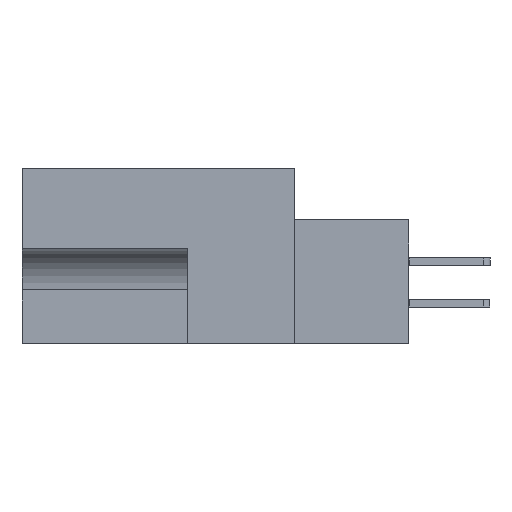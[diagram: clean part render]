
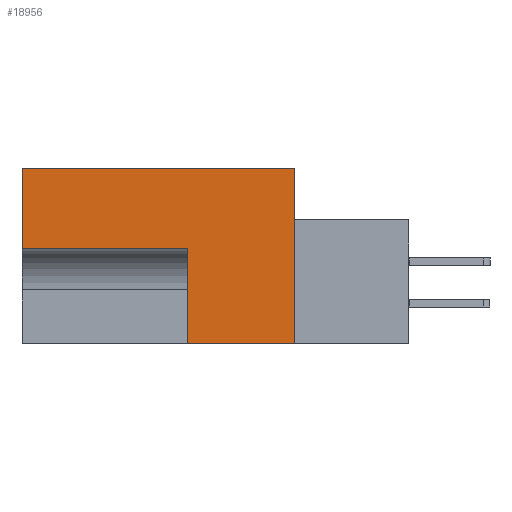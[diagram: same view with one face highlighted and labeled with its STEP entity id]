
A CAD part, left-side view. The second image highlights one B-rep face of the part: STEP entity #18956.
In plain terms, the highlighted planar face has unit normal (-1, 0, 0).
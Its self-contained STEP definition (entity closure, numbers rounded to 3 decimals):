
#2297 = EDGE_CURVE ( 'NONE', #13892, #23138, #31262, .T. ) ;
#3985 = VERTEX_POINT ( 'NONE', #21897 ) ;
#4034 = CARTESIAN_POINT ( 'NONE',  ( 0., 20.955, -13.487 ) ) ;
#5155 = DIRECTION ( 'NONE',  ( 0., 0., -1. ) ) ;
#5319 = DIRECTION ( 'NONE',  ( 0., 0., 1. ) ) ;
#7769 = CARTESIAN_POINT ( 'NONE',  ( 0., 0., 0. ) ) ;
#9452 = EDGE_CURVE ( 'NONE', #26596, #13892, #23545, .T. ) ;
#11130 = ORIENTED_EDGE ( 'NONE', *, *, #23562, .F. ) ;
#11263 = ORIENTED_EDGE ( 'NONE', *, *, #2297, .F. ) ;
#11365 = VECTOR ( 'NONE', #5319, 1000. ) ;
#11494 = VECTOR ( 'NONE', #23254, 1000. ) ;
#11643 = CARTESIAN_POINT ( 'NONE',  ( 0., 11.506, 0. ) ) ;
#11951 = PLANE ( 'NONE',  #33710 ) ;
#13275 = VECTOR ( 'NONE', #32747, 1000. ) ;
#13278 = VERTEX_POINT ( 'NONE', #27387 ) ;
#13892 = VERTEX_POINT ( 'NONE', #7769 ) ;
#14744 = DIRECTION ( 'NONE',  ( 0., -1., 0. ) ) ;
#16307 = CARTESIAN_POINT ( 'NONE',  ( 0., 0., 0. ) ) ;
#16682 = LINE ( 'NONE', #27298, #13275 ) ;
#17505 = LINE ( 'NONE', #4034, #11494 ) ;
#17528 = DIRECTION ( 'NONE',  ( 0., 1., 0. ) ) ;
#18627 = ORIENTED_EDGE ( 'NONE', *, *, #25774, .F. ) ;
#18727 = CARTESIAN_POINT ( 'NONE',  ( 0., 20.955, 0. ) ) ;
#18956 = ADVANCED_FACE ( 'NONE', ( #33670 ), #11951, .F. ) ;
#19690 = VECTOR ( 'NONE', #17528, 1000. ) ;
#20861 = CARTESIAN_POINT ( 'NONE',  ( 0., 0., -13.487 ) ) ;
#21897 = CARTESIAN_POINT ( 'NONE',  ( 0., 8.255, -6.172 ) ) ;
#22551 = DIRECTION ( 'NONE',  ( 0., 0., -1. ) ) ;
#22715 = CARTESIAN_POINT ( 'NONE',  ( 0., 8.255, -6.172 ) ) ;
#23138 = VERTEX_POINT ( 'NONE', #20861 ) ;
#23254 = DIRECTION ( 'NONE',  ( 0., 0., 1. ) ) ;
#23545 = LINE ( 'NONE', #11643, #29469 ) ;
#23562 = EDGE_CURVE ( 'NONE', #3985, #13278, #26935, .T. ) ;
#23663 = CARTESIAN_POINT ( 'NONE',  ( 0., 8.255, -13.487 ) ) ;
#25774 = EDGE_CURVE ( 'NONE', #29394, #3985, #28055, .T. ) ;
#26596 = VERTEX_POINT ( 'NONE', #18727 ) ;
#26605 = EDGE_LOOP ( 'NONE', ( #33394, #11263, #27914, #29822, #11130, #18627 ) ) ;
#26935 = LINE ( 'NONE', #22715, #19690 ) ;
#27298 = CARTESIAN_POINT ( 'NONE',  ( 0., -8.814, -13.487 ) ) ;
#27387 = CARTESIAN_POINT ( 'NONE',  ( 0., 20.955, -6.172 ) ) ;
#27914 = ORIENTED_EDGE ( 'NONE', *, *, #9452, .F. ) ;
#28055 = LINE ( 'NONE', #23663, #11365 ) ;
#28235 = DIRECTION ( 'NONE',  ( 1., 0., 0. ) ) ;
#29394 = VERTEX_POINT ( 'NONE', #30460 ) ;
#29469 = VECTOR ( 'NONE', #14744, 1000. ) ;
#29822 = ORIENTED_EDGE ( 'NONE', *, *, #31658, .F. ) ;
#30319 = EDGE_CURVE ( 'NONE', #23138, #29394, #16682, .T. ) ;
#30460 = CARTESIAN_POINT ( 'NONE',  ( 0., 8.255, -13.487 ) ) ;
#30851 = CARTESIAN_POINT ( 'NONE',  ( 0., 0., 0. ) ) ;
#31262 = LINE ( 'NONE', #16307, #31685 ) ;
#31658 = EDGE_CURVE ( 'NONE', #13278, #26596, #17505, .T. ) ;
#31685 = VECTOR ( 'NONE', #5155, 1000. ) ;
#32747 = DIRECTION ( 'NONE',  ( 0., 1., 0. ) ) ;
#33394 = ORIENTED_EDGE ( 'NONE', *, *, #30319, .F. ) ;
#33670 = FACE_OUTER_BOUND ( 'NONE', #26605, .T. ) ;
#33710 = AXIS2_PLACEMENT_3D ( 'NONE', #30851, #28235, #22551 ) ;
